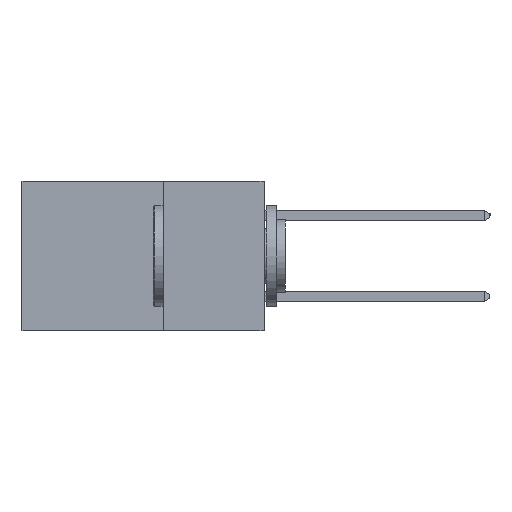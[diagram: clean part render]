
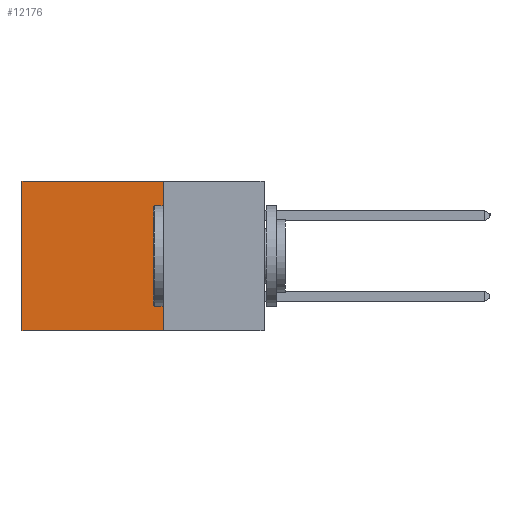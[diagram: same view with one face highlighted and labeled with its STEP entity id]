
A CAD part, left-side view. The second image highlights one B-rep face of the part: STEP entity #12176.
In plain terms, the highlighted planar face has unit normal (-1, 0, 0).
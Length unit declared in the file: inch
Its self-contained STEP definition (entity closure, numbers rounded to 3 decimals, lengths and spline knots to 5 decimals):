
#127 = LINE ( 'NONE', #4251, #3051 ) ;
#646 = VERTEX_POINT ( 'NONE', #11343 ) ;
#699 = FACE_OUTER_BOUND ( 'NONE', #5991, .T. ) ;
#1271 = ORIENTED_EDGE ( 'NONE', *, *, #5726, .T. ) ;
#1306 = EDGE_CURVE ( 'NONE', #8049, #646, #1738, .T. ) ;
#1738 = LINE ( 'NONE', #4788, #10413 ) ;
#2077 = VECTOR ( 'NONE', #10675, 39.37008 ) ;
#2305 = LINE ( 'NONE', #5154, #4079 ) ;
#2490 = ORIENTED_EDGE ( 'NONE', *, *, #1306, .F. ) ;
#3051 = VECTOR ( 'NONE', #9235, 39.37008 ) ;
#3370 = AXIS2_PLACEMENT_3D ( 'NONE', #9807, #6724, #4839 ) ;
#4079 = VECTOR ( 'NONE', #9242, 39.37008 ) ;
#4251 = CARTESIAN_POINT ( 'NONE',  ( 0.2615, 0.6, -0.37 ) ) ;
#4402 = CARTESIAN_POINT ( 'NONE',  ( 0.2615, 0.25, 0. ) ) ;
#4788 = CARTESIAN_POINT ( 'NONE',  ( 0.2615, 0.25, -0.37 ) ) ;
#4839 = DIRECTION ( 'NONE',  ( 0., 0., -1. ) ) ;
#5154 = CARTESIAN_POINT ( 'NONE',  ( 0.2615, 0.25, -0.37 ) ) ;
#5548 = CARTESIAN_POINT ( 'NONE',  ( 0.2615, 0.6, -0.37 ) ) ;
#5553 = ORIENTED_EDGE ( 'NONE', *, *, #8239, .T. ) ;
#5726 = EDGE_CURVE ( 'NONE', #8049, #12435, #12621, .T. ) ;
#5991 = EDGE_LOOP ( 'NONE', ( #5553, #6039, #2490, #1271 ) ) ;
#6039 = ORIENTED_EDGE ( 'NONE', *, *, #11031, .F. ) ;
#6724 = DIRECTION ( 'NONE',  ( 1., 0., 0. ) ) ;
#6890 = CARTESIAN_POINT ( 'NONE',  ( 0.2615, 0.25, 0. ) ) ;
#7495 = VERTEX_POINT ( 'NONE', #5548 ) ;
#7849 = PLANE ( 'NONE',  #3370 ) ;
#8049 = VERTEX_POINT ( 'NONE', #6890 ) ;
#8239 = EDGE_CURVE ( 'NONE', #12435, #7495, #127, .T. ) ;
#8941 = DIRECTION ( 'NONE',  ( 0., 0., -1. ) ) ;
#9235 = DIRECTION ( 'NONE',  ( 0., 0., -1. ) ) ;
#9242 = DIRECTION ( 'NONE',  ( 0., 1., 0. ) ) ;
#9807 = CARTESIAN_POINT ( 'NONE',  ( 0.2615, 0.25, -0.37 ) ) ;
#10413 = VECTOR ( 'NONE', #8941, 39.37008 ) ;
#10675 = DIRECTION ( 'NONE',  ( 0., 1., 0. ) ) ;
#11031 = EDGE_CURVE ( 'NONE', #646, #7495, #2305, .T. ) ;
#11343 = CARTESIAN_POINT ( 'NONE',  ( 0.2615, 0.25, -0.37 ) ) ;
#12176 = ADVANCED_FACE ( 'NONE', ( #699 ), #7849, .F. ) ;
#12282 = CARTESIAN_POINT ( 'NONE',  ( 0.2615, 0.6, 0. ) ) ;
#12435 = VERTEX_POINT ( 'NONE', #12282 ) ;
#12621 = LINE ( 'NONE', #4402, #2077 ) ;
